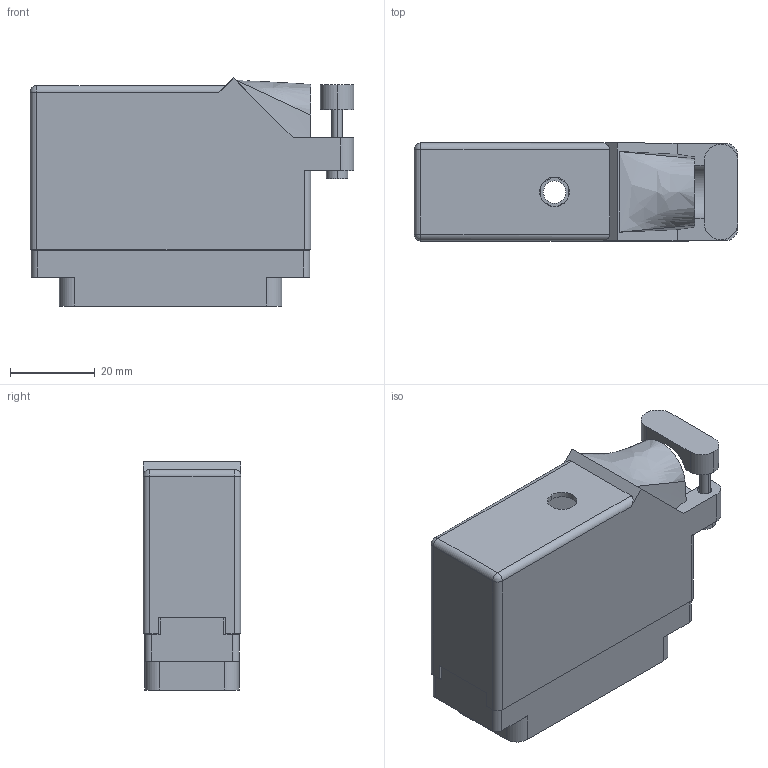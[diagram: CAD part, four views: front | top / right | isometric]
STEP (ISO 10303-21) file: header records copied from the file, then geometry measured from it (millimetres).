
FILE_DESCRIPTION (( 'STEP AP203' ), '1' );
FILE_NAME ('516-056-500-520.STEP', '2020-03-10T06:58:44', ( '' ), ( '' ), 'SwSTEP 2.0', 'SolidWorks 2016', '' );
FILE_SCHEMA (( 'CONFIG_CONTROL_DESIGN' ));
Length unit declared in the file: inch
Products named in the file (4): 516-230-001_Plastic - 056 Side Entry; 516 Plug Insulator_056; 516-292-001_500 Contact; 516-056-500-520
Assembly tree (58 placements, depth 2):
  516-056-500-520
    516 Plug Insulator_056
    516-292-001_500 Contact  x56
    516-230-001_Plastic - 056 Side Entry
Bounding box: 76.5 x 23.11 x 53.92 mm (x, y, z)
Volume: 25747.5 mm3; surface area: 42480.8 mm2
Topology: 58 solids, 58 shells, 5545 faces, 16104 edges, 10694 vertices
Faces by surface type: plane 3342, cylinder 1860, bspline 339, cone 2, sphere 2
Entity records: 48002 total; most frequent: CARTESIAN_POINT 8470, ORIENTED_EDGE 8004, DIRECTION 7763, EDGE_CURVE 4002, VECTOR 2999, LINE 2999, VERTEX_POINT 2664, AXIS2_PLACEMENT_3D 2382
